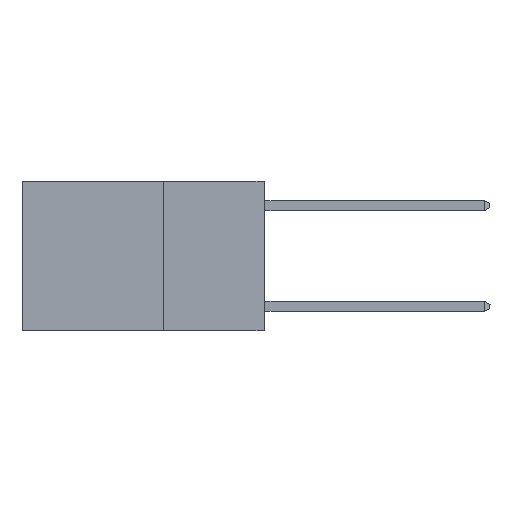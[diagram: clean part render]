
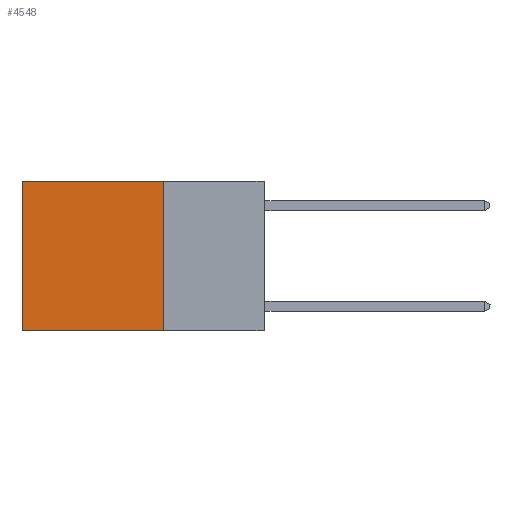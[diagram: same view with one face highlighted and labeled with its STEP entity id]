
A CAD part, left-side view. The second image highlights one B-rep face of the part: STEP entity #4548.
In plain terms, the highlighted planar face has unit normal (-1, 0, 0).
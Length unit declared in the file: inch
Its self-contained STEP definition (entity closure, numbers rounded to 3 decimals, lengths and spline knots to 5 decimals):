
#26 = VERTEX_POINT ( 'NONE', #2497 ) ;
#200 = VERTEX_POINT ( 'NONE', #3560 ) ;
#330 = AXIS2_PLACEMENT_3D ( 'NONE', #2305, #5632, #12900 ) ;
#637 = EDGE_CURVE ( 'NONE', #13190, #26, #3124, .T. ) ;
#1011 = ORIENTED_EDGE ( 'NONE', *, *, #13286, .F. ) ;
#1740 = CARTESIAN_POINT ( 'NONE',  ( 0.2625, 0.25, 0. ) ) ;
#1855 = EDGE_CURVE ( 'NONE', #26, #200, #3990, .T. ) ;
#2305 = CARTESIAN_POINT ( 'NONE',  ( 0.2625, 0.25, 0. ) ) ;
#2497 = CARTESIAN_POINT ( 'NONE',  ( 0.2625, 0.6, 0. ) ) ;
#3124 = LINE ( 'NONE', #1740, #13907 ) ;
#3560 = CARTESIAN_POINT ( 'NONE',  ( 0.2625, 0.6, -0.37 ) ) ;
#3590 = ORIENTED_EDGE ( 'NONE', *, *, #5412, .F. ) ;
#3764 = DIRECTION ( 'NONE',  ( 0., 1., 0. ) ) ;
#3990 = LINE ( 'NONE', #8895, #12014 ) ;
#4145 = LINE ( 'NONE', #5015, #6651 ) ;
#4353 = CARTESIAN_POINT ( 'NONE',  ( 0.2625, 0.25, -0.37 ) ) ;
#4548 = ADVANCED_FACE ( 'NONE', ( #6338 ), #4561, .F. ) ;
#4561 = PLANE ( 'NONE',  #330 ) ;
#5015 = CARTESIAN_POINT ( 'NONE',  ( 0.2625, 0.25, 0. ) ) ;
#5298 = VECTOR ( 'NONE', #3764, 39.37008 ) ;
#5302 = ORIENTED_EDGE ( 'NONE', *, *, #637, .T. ) ;
#5412 = EDGE_CURVE ( 'NONE', #13190, #5674, #4145, .T. ) ;
#5632 = DIRECTION ( 'NONE',  ( 1., 0., 0. ) ) ;
#5674 = VERTEX_POINT ( 'NONE', #4353 ) ;
#6086 = DIRECTION ( 'NONE',  ( 0., 0., -1. ) ) ;
#6338 = FACE_OUTER_BOUND ( 'NONE', #9018, .T. ) ;
#6651 = VECTOR ( 'NONE', #6086, 39.37008 ) ;
#7636 = ORIENTED_EDGE ( 'NONE', *, *, #1855, .T. ) ;
#7865 = DIRECTION ( 'NONE',  ( 0., 0., -1. ) ) ;
#8895 = CARTESIAN_POINT ( 'NONE',  ( 0.2625, 0.6, 0. ) ) ;
#9018 = EDGE_LOOP ( 'NONE', ( #7636, #1011, #3590, #5302 ) ) ;
#9084 = CARTESIAN_POINT ( 'NONE',  ( 0.2625, 0.25, -0.37 ) ) ;
#10627 = LINE ( 'NONE', #9084, #5298 ) ;
#10801 = DIRECTION ( 'NONE',  ( 0., 1., 0. ) ) ;
#12014 = VECTOR ( 'NONE', #7865, 39.37008 ) ;
#12900 = DIRECTION ( 'NONE',  ( 0., 0., -1. ) ) ;
#12987 = CARTESIAN_POINT ( 'NONE',  ( 0.2625, 0.25, 0. ) ) ;
#13190 = VERTEX_POINT ( 'NONE', #12987 ) ;
#13286 = EDGE_CURVE ( 'NONE', #5674, #200, #10627, .T. ) ;
#13907 = VECTOR ( 'NONE', #10801, 39.37008 ) ;
